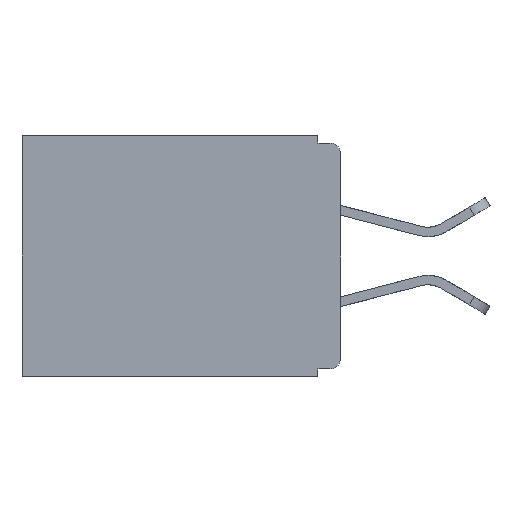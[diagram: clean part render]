
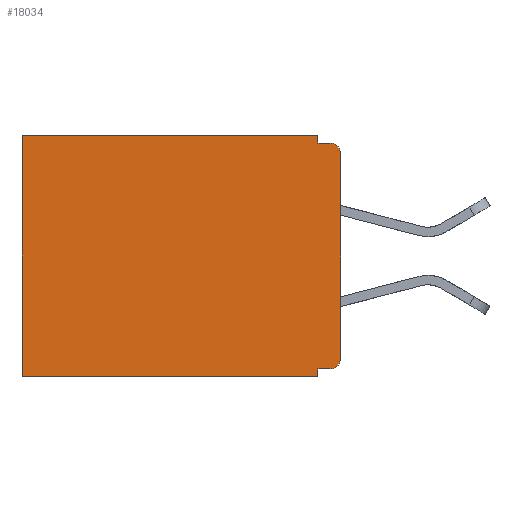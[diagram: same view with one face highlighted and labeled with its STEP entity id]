
A CAD part, left-side view. The second image highlights one B-rep face of the part: STEP entity #18034.
In plain terms, the highlighted planar face has unit normal (-1, 0, 0).
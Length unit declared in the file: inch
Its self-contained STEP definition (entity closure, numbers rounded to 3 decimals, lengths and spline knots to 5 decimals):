
#590 = AXIS2_PLACEMENT_3D ( 'NONE', #13731, #10821, #10465 ) ;
#662 = CARTESIAN_POINT ( 'NONE',  ( 0.3, 0.031, -0.33 ) ) ;
#949 = ORIENTED_EDGE ( 'NONE', *, *, #21695, .F. ) ;
#1316 = CARTESIAN_POINT ( 'NONE',  ( 0.3, 0.031, -0.32 ) ) ;
#1422 = PLANE ( 'NONE',  #10202 ) ;
#1501 = DIRECTION ( 'NONE',  ( 1., 0., 0. ) ) ;
#1657 = EDGE_CURVE ( 'NONE', #12760, #20115, #14423, .T. ) ;
#1661 = ORIENTED_EDGE ( 'NONE', *, *, #16418, .F. ) ;
#1843 = LINE ( 'NONE', #23226, #11382 ) ;
#2061 = CARTESIAN_POINT ( 'NONE',  ( 0.3, 0., -0.025 ) ) ;
#2351 = DIRECTION ( 'NONE',  ( 0., -1., 0. ) ) ;
#2520 = EDGE_CURVE ( 'NONE', #10245, #20964, #14381, .T. ) ;
#2849 = VECTOR ( 'NONE', #12159, 39.37008 ) ;
#3537 = ORIENTED_EDGE ( 'NONE', *, *, #9884, .T. ) ;
#3700 = VECTOR ( 'NONE', #12481, 39.37008 ) ;
#4509 = EDGE_LOOP ( 'NONE', ( #21725, #15934, #949, #23964, #23405, #3537, #6691, #1661, #10618, #19834 ) ) ;
#5116 = DIRECTION ( 'NONE',  ( 0., 1., 0. ) ) ;
#5819 = LINE ( 'NONE', #12005, #15282 ) ;
#6691 = ORIENTED_EDGE ( 'NONE', *, *, #22243, .F. ) ;
#7886 = CARTESIAN_POINT ( 'NONE',  ( 0.3, 0.015, -0.01 ) ) ;
#8097 = VECTOR ( 'NONE', #5116, 39.37008 ) ;
#8227 = VECTOR ( 'NONE', #23479, 39.37008 ) ;
#8349 = AXIS2_PLACEMENT_3D ( 'NONE', #18273, #18533, #20649 ) ;
#8824 = DIRECTION ( 'NONE',  ( 0., 0., -1. ) ) ;
#8873 = EDGE_CURVE ( 'NONE', #12760, #18638, #21808, .T. ) ;
#9571 = VERTEX_POINT ( 'NONE', #16820 ) ;
#9786 = CARTESIAN_POINT ( 'NONE',  ( 0.3, 0.031, 0. ) ) ;
#9884 = EDGE_CURVE ( 'NONE', #18574, #9893, #1843, .T. ) ;
#9893 = VERTEX_POINT ( 'NONE', #17849 ) ;
#10202 = AXIS2_PLACEMENT_3D ( 'NONE', #12860, #1501, #14708 ) ;
#10245 = VERTEX_POINT ( 'NONE', #2061 ) ;
#10465 = DIRECTION ( 'NONE',  ( 0., 0., -1. ) ) ;
#10618 = ORIENTED_EDGE ( 'NONE', *, *, #8873, .F. ) ;
#10622 = LINE ( 'NONE', #18001, #14412 ) ;
#10821 = DIRECTION ( 'NONE',  ( -1., 0., 0. ) ) ;
#11382 = VECTOR ( 'NONE', #19618, 39.37008 ) ;
#12005 = CARTESIAN_POINT ( 'NONE',  ( 0.3, 0., -0.01 ) ) ;
#12159 = DIRECTION ( 'NONE',  ( 0., 1., 0. ) ) ;
#12481 = DIRECTION ( 'NONE',  ( 0., 0., -1. ) ) ;
#12760 = VERTEX_POINT ( 'NONE', #15948 ) ;
#12860 = CARTESIAN_POINT ( 'NONE',  ( 0.3, 0., -0.33 ) ) ;
#12949 = LINE ( 'NONE', #19461, #2849 ) ;
#13174 = CARTESIAN_POINT ( 'NONE',  ( 0.3, 0., -0.32 ) ) ;
#13247 = LINE ( 'NONE', #19713, #8227 ) ;
#13477 = EDGE_CURVE ( 'NONE', #14344, #18574, #18562, .T. ) ;
#13731 = CARTESIAN_POINT ( 'NONE',  ( 0.3, 0.015, -0.025 ) ) ;
#14344 = VERTEX_POINT ( 'NONE', #9786 ) ;
#14381 = CIRCLE ( 'NONE', #590, 0.015 ) ;
#14412 = VECTOR ( 'NONE', #8824, 39.37008 ) ;
#14423 = CIRCLE ( 'NONE', #8349, 0.015 ) ;
#14708 = DIRECTION ( 'NONE',  ( 0., 0., -1. ) ) ;
#15282 = VECTOR ( 'NONE', #2351, 39.37008 ) ;
#15934 = ORIENTED_EDGE ( 'NONE', *, *, #2520, .T. ) ;
#15948 = CARTESIAN_POINT ( 'NONE',  ( 0.3, 0.015, -0.32 ) ) ;
#16327 = CARTESIAN_POINT ( 'NONE',  ( 0.3, 0., 0. ) ) ;
#16418 = EDGE_CURVE ( 'NONE', #18638, #19798, #13247, .T. ) ;
#16424 = EDGE_CURVE ( 'NONE', #10245, #20115, #18110, .T. ) ;
#16820 = CARTESIAN_POINT ( 'NONE',  ( 0.3, 0.031, -0.01 ) ) ;
#16909 = VECTOR ( 'NONE', #18713, 39.37008 ) ;
#16921 = FACE_OUTER_BOUND ( 'NONE', #4509, .T. ) ;
#17849 = CARTESIAN_POINT ( 'NONE',  ( 0.3, 0.437, -0.33 ) ) ;
#18001 = CARTESIAN_POINT ( 'NONE',  ( 0.3, 0.031, 0. ) ) ;
#18034 = ADVANCED_FACE ( 'NONE', ( #16921 ), #1422, .F. ) ;
#18110 = LINE ( 'NONE', #21648, #3700 ) ;
#18273 = CARTESIAN_POINT ( 'NONE',  ( 0.3, 0.015, -0.305 ) ) ;
#18533 = DIRECTION ( 'NONE',  ( -1., 0., 0. ) ) ;
#18562 = LINE ( 'NONE', #16327, #8097 ) ;
#18574 = VERTEX_POINT ( 'NONE', #19898 ) ;
#18638 = VERTEX_POINT ( 'NONE', #1316 ) ;
#18713 = DIRECTION ( 'NONE',  ( 0., 1., 0. ) ) ;
#19461 = CARTESIAN_POINT ( 'NONE',  ( 0.3, 0., -0.33 ) ) ;
#19618 = DIRECTION ( 'NONE',  ( 0., 0., -1. ) ) ;
#19713 = CARTESIAN_POINT ( 'NONE',  ( 0.3, 0.031, -0.33 ) ) ;
#19798 = VERTEX_POINT ( 'NONE', #662 ) ;
#19834 = ORIENTED_EDGE ( 'NONE', *, *, #1657, .T. ) ;
#19898 = CARTESIAN_POINT ( 'NONE',  ( 0.3, 0.437, 0. ) ) ;
#20115 = VERTEX_POINT ( 'NONE', #22177 ) ;
#20649 = DIRECTION ( 'NONE',  ( 0., 0., -1. ) ) ;
#20964 = VERTEX_POINT ( 'NONE', #7886 ) ;
#21648 = CARTESIAN_POINT ( 'NONE',  ( 0.3, 0., -0.33 ) ) ;
#21695 = EDGE_CURVE ( 'NONE', #9571, #20964, #5819, .T. ) ;
#21725 = ORIENTED_EDGE ( 'NONE', *, *, #16424, .F. ) ;
#21808 = LINE ( 'NONE', #13174, #16909 ) ;
#22177 = CARTESIAN_POINT ( 'NONE',  ( 0.3, 0., -0.305 ) ) ;
#22243 = EDGE_CURVE ( 'NONE', #19798, #9893, #12949, .T. ) ;
#22422 = EDGE_CURVE ( 'NONE', #14344, #9571, #10622, .T. ) ;
#23226 = CARTESIAN_POINT ( 'NONE',  ( 0.3, 0.437, -0.33 ) ) ;
#23405 = ORIENTED_EDGE ( 'NONE', *, *, #13477, .T. ) ;
#23479 = DIRECTION ( 'NONE',  ( 0., 0., -1. ) ) ;
#23964 = ORIENTED_EDGE ( 'NONE', *, *, #22422, .F. ) ;
